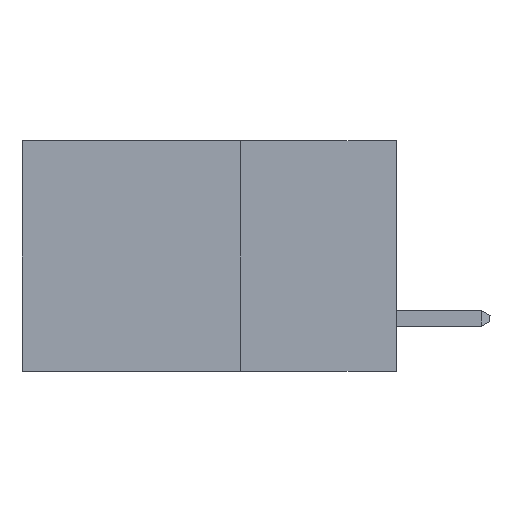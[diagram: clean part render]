
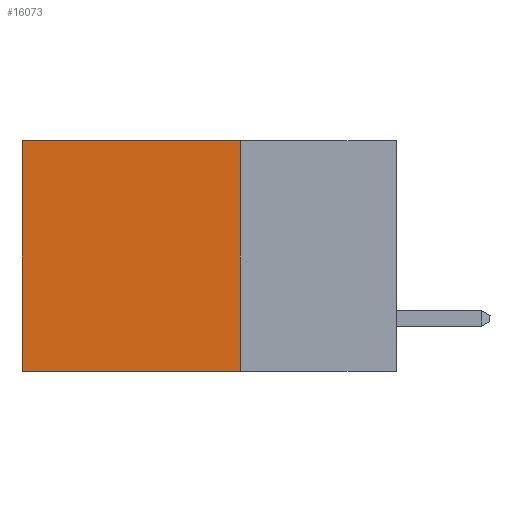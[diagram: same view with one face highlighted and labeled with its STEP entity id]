
A CAD part, left-side view. The second image highlights one B-rep face of the part: STEP entity #16073.
In plain terms, the highlighted planar face has unit normal (-1, 0, 0).
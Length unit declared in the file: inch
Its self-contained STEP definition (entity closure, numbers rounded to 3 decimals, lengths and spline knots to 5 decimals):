
#636 = EDGE_CURVE ( 'NONE', #7646, #16970, #17492, .T. ) ;
#783 = DIRECTION ( 'NONE',  ( 0., 0., -1. ) ) ;
#2333 = CARTESIAN_POINT ( 'NONE',  ( 0.2615, 0.6, 0. ) ) ;
#2427 = VECTOR ( 'NONE', #14109, 39.37008 ) ;
#2623 = DIRECTION ( 'NONE',  ( 0., 1., 0. ) ) ;
#3501 = EDGE_LOOP ( 'NONE', ( #6222, #17807, #19927, #11482 ) ) ;
#3627 = CARTESIAN_POINT ( 'NONE',  ( 0.2615, 0.6, -0.37 ) ) ;
#3739 = LINE ( 'NONE', #10404, #2427 ) ;
#4260 = CARTESIAN_POINT ( 'NONE',  ( 0.2615, 0.25, 0. ) ) ;
#4505 = LINE ( 'NONE', #12705, #9443 ) ;
#4681 = CARTESIAN_POINT ( 'NONE',  ( 0.2615, 0.25, 0. ) ) ;
#5770 = VERTEX_POINT ( 'NONE', #20671 ) ;
#6222 = ORIENTED_EDGE ( 'NONE', *, *, #11334, .T. ) ;
#7431 = DIRECTION ( 'NONE',  ( 0., 0., -1. ) ) ;
#7541 = CARTESIAN_POINT ( 'NONE',  ( 0.2615, 0.25, -0.37 ) ) ;
#7646 = VERTEX_POINT ( 'NONE', #4681 ) ;
#8810 = AXIS2_PLACEMENT_3D ( 'NONE', #7541, #10704, #7431 ) ;
#9443 = VECTOR ( 'NONE', #19380, 39.37008 ) ;
#10404 = CARTESIAN_POINT ( 'NONE',  ( 0.2615, 0.6, -0.37 ) ) ;
#10704 = DIRECTION ( 'NONE',  ( 1., 0., 0. ) ) ;
#10918 = PLANE ( 'NONE',  #8810 ) ;
#11311 = EDGE_CURVE ( 'NONE', #7646, #5770, #17191, .T. ) ;
#11334 = EDGE_CURVE ( 'NONE', #16970, #17285, #3739, .T. ) ;
#11482 = ORIENTED_EDGE ( 'NONE', *, *, #636, .T. ) ;
#12358 = FACE_OUTER_BOUND ( 'NONE', #3501, .T. ) ;
#12705 = CARTESIAN_POINT ( 'NONE',  ( 0.2615, 0.25, -0.37 ) ) ;
#14109 = DIRECTION ( 'NONE',  ( 0., 0., -1. ) ) ;
#14588 = EDGE_CURVE ( 'NONE', #5770, #17285, #4505, .T. ) ;
#15703 = VECTOR ( 'NONE', #783, 39.37008 ) ;
#15767 = CARTESIAN_POINT ( 'NONE',  ( 0.2615, 0.25, -0.37 ) ) ;
#16073 = ADVANCED_FACE ( 'NONE', ( #12358 ), #10918, .F. ) ;
#16970 = VERTEX_POINT ( 'NONE', #2333 ) ;
#17191 = LINE ( 'NONE', #15767, #15703 ) ;
#17285 = VERTEX_POINT ( 'NONE', #3627 ) ;
#17492 = LINE ( 'NONE', #4260, #19852 ) ;
#17807 = ORIENTED_EDGE ( 'NONE', *, *, #14588, .F. ) ;
#19380 = DIRECTION ( 'NONE',  ( 0., 1., 0. ) ) ;
#19852 = VECTOR ( 'NONE', #2623, 39.37008 ) ;
#19927 = ORIENTED_EDGE ( 'NONE', *, *, #11311, .F. ) ;
#20671 = CARTESIAN_POINT ( 'NONE',  ( 0.2615, 0.25, -0.37 ) ) ;
